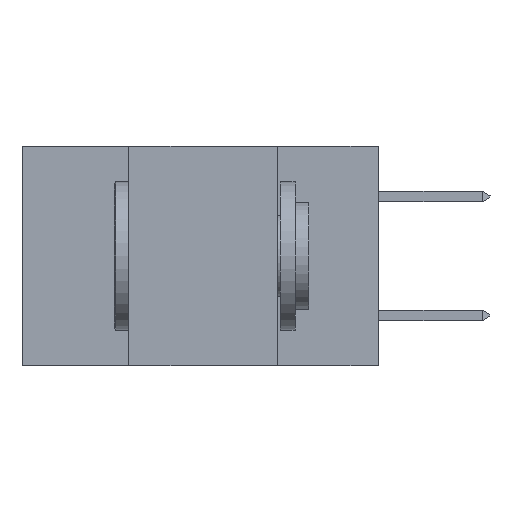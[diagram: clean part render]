
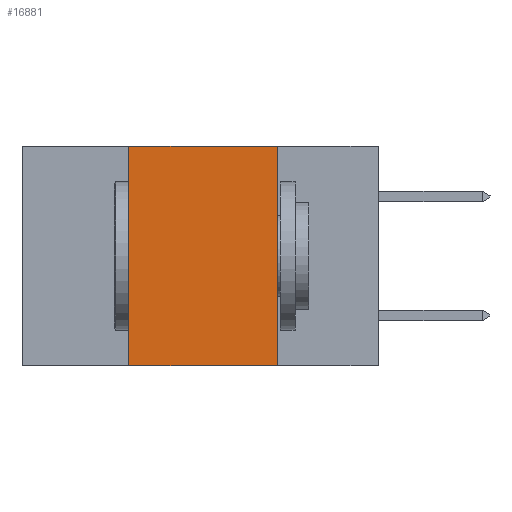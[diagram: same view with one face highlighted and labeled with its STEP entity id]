
A CAD part, left-side view. The second image highlights one B-rep face of the part: STEP entity #16881.
In plain terms, the highlighted planar face has unit normal (-1, 0, 0).
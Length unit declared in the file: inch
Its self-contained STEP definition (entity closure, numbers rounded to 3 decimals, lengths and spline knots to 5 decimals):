
#140 = CARTESIAN_POINT ( 'NONE',  ( 0., 0.42, -0.37 ) ) ;
#579 = DIRECTION ( 'NONE',  ( 0., 0., 1. ) ) ;
#608 = EDGE_CURVE ( 'NONE', #4877, #3908, #11311, .T. ) ;
#1123 = VECTOR ( 'NONE', #6133, 39.37008 ) ;
#2115 = CARTESIAN_POINT ( 'NONE',  ( 0., 0.6, 0. ) ) ;
#3077 = ORIENTED_EDGE ( 'NONE', *, *, #9195, .F. ) ;
#3908 = VERTEX_POINT ( 'NONE', #6880 ) ;
#4183 = LINE ( 'NONE', #12682, #26076 ) ;
#4877 = VERTEX_POINT ( 'NONE', #140 ) ;
#5547 = EDGE_CURVE ( 'NONE', #26952, #26863, #22829, .T. ) ;
#6051 = EDGE_CURVE ( 'NONE', #4877, #26863, #10624, .T. ) ;
#6133 = DIRECTION ( 'NONE',  ( 0., -1., 0. ) ) ;
#6880 = CARTESIAN_POINT ( 'NONE',  ( 0., 0.42, 0. ) ) ;
#8414 = DIRECTION ( 'NONE',  ( 0., 0., -1. ) ) ;
#8685 = CARTESIAN_POINT ( 'NONE',  ( 0., 0.17, -0.37 ) ) ;
#9092 = EDGE_LOOP ( 'NONE', ( #14601, #3077, #23271, #11655 ) ) ;
#9195 = EDGE_CURVE ( 'NONE', #3908, #26952, #4183, .T. ) ;
#10624 = LINE ( 'NONE', #12825, #1123 ) ;
#11311 = LINE ( 'NONE', #13669, #11940 ) ;
#11655 = ORIENTED_EDGE ( 'NONE', *, *, #6051, .T. ) ;
#11940 = VECTOR ( 'NONE', #579, 39.37008 ) ;
#12435 = DIRECTION ( 'NONE',  ( 1., 0., 0. ) ) ;
#12682 = CARTESIAN_POINT ( 'NONE',  ( 0., 0.6, 0. ) ) ;
#12825 = CARTESIAN_POINT ( 'NONE',  ( 0., 0.6, -0.37 ) ) ;
#13669 = CARTESIAN_POINT ( 'NONE',  ( 0., 0.42, -0.37 ) ) ;
#13886 = AXIS2_PLACEMENT_3D ( 'NONE', #2115, #12435, #23224 ) ;
#14601 = ORIENTED_EDGE ( 'NONE', *, *, #5547, .F. ) ;
#14897 = DIRECTION ( 'NONE',  ( 0., -1., 0. ) ) ;
#14912 = FACE_OUTER_BOUND ( 'NONE', #9092, .T. ) ;
#16881 = ADVANCED_FACE ( 'NONE', ( #14912 ), #18799, .F. ) ;
#18799 = PLANE ( 'NONE',  #13886 ) ;
#19819 = CARTESIAN_POINT ( 'NONE',  ( 0., 0.17, -0.37 ) ) ;
#22829 = LINE ( 'NONE', #8685, #25506 ) ;
#23095 = CARTESIAN_POINT ( 'NONE',  ( 0., 0.17, 0. ) ) ;
#23224 = DIRECTION ( 'NONE',  ( 0., 0., -1. ) ) ;
#23271 = ORIENTED_EDGE ( 'NONE', *, *, #608, .F. ) ;
#25506 = VECTOR ( 'NONE', #8414, 39.37008 ) ;
#26076 = VECTOR ( 'NONE', #14897, 39.37008 ) ;
#26863 = VERTEX_POINT ( 'NONE', #19819 ) ;
#26952 = VERTEX_POINT ( 'NONE', #23095 ) ;
